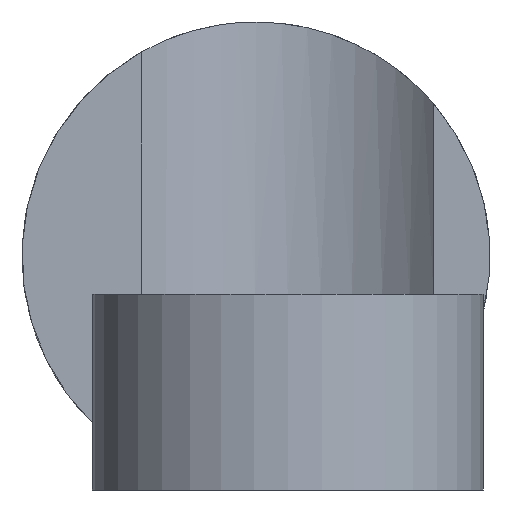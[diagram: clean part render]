
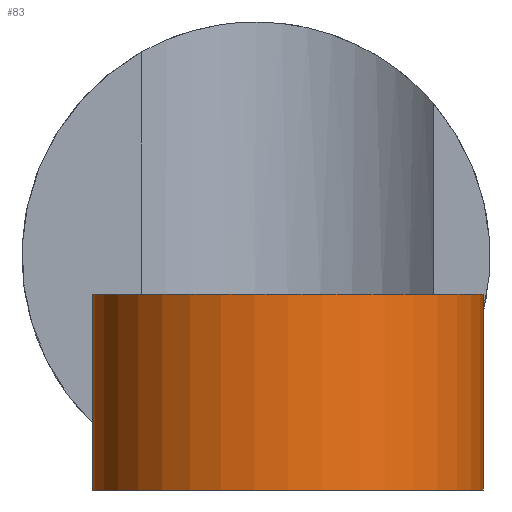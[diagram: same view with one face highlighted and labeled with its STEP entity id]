
A CAD part, left-side view. The second image highlights one B-rep face of the part: STEP entity #83.
In plain terms, the highlighted cylindrical face has radius 6 mm (diameter 12 mm), a partial arc.
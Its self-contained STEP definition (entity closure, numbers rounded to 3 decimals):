
#21 = DIRECTION ( 'NONE',  ( 0., 0., -1. ) ) ;
#33 = DIRECTION ( 'NONE',  ( 0., 0., 1. ) ) ;
#43 = CARTESIAN_POINT ( 'NONE',  ( -17.5, 0., 6. ) ) ;
#61 = ORIENTED_EDGE ( 'NONE', *, *, #650, .F. ) ;
#64 = EDGE_CURVE ( 'NONE', #550, #421, #157, .T. ) ;
#72 = AXIS2_PLACEMENT_3D ( 'NONE', #43, #623, #237 ) ;
#83 = ADVANCED_FACE ( 'NONE', ( #720 ), #537, .T. ) ;
#84 = CARTESIAN_POINT ( 'NONE',  ( -17.5, -6., 0. ) ) ;
#95 = CARTESIAN_POINT ( 'NONE',  ( -17.5, 0., 0. ) ) ;
#115 = CARTESIAN_POINT ( 'NONE',  ( -17.5, 6., 0. ) ) ;
#157 = LINE ( 'NONE', #440, #447 ) ;
#236 = AXIS2_PLACEMENT_3D ( 'NONE', #656, #21, #489 ) ;
#237 = DIRECTION ( 'NONE',  ( -1., 0., 0. ) ) ;
#262 = CIRCLE ( 'NONE', #236, 6. ) ;
#264 = EDGE_CURVE ( 'NONE', #421, #706, #500, .T. ) ;
#285 = VECTOR ( 'NONE', #33, 1000. ) ;
#325 = AXIS2_PLACEMENT_3D ( 'NONE', #95, #665, #496 ) ;
#397 = ORIENTED_EDGE ( 'NONE', *, *, #264, .T. ) ;
#413 = VERTEX_POINT ( 'NONE', #115 ) ;
#421 = VERTEX_POINT ( 'NONE', #530 ) ;
#440 = CARTESIAN_POINT ( 'NONE',  ( -17.5, -6., 0. ) ) ;
#447 = VECTOR ( 'NONE', #609, 1000. ) ;
#489 = DIRECTION ( 'NONE',  ( -1., 0., 0. ) ) ;
#496 = DIRECTION ( 'NONE',  ( 1., 0., 0. ) ) ;
#500 = CIRCLE ( 'NONE', #72, 6. ) ;
#530 = CARTESIAN_POINT ( 'NONE',  ( -17.5, -6., 6. ) ) ;
#534 = CARTESIAN_POINT ( 'NONE',  ( -17.5, 6., 0. ) ) ;
#537 = CYLINDRICAL_SURFACE ( 'NONE', #325, 6. ) ;
#550 = VERTEX_POINT ( 'NONE', #84 ) ;
#555 = EDGE_CURVE ( 'NONE', #550, #413, #262, .T. ) ;
#557 = LINE ( 'NONE', #534, #285 ) ;
#589 = ORIENTED_EDGE ( 'NONE', *, *, #64, .T. ) ;
#609 = DIRECTION ( 'NONE',  ( 0., 0., 1. ) ) ;
#623 = DIRECTION ( 'NONE',  ( 0., 0., -1. ) ) ;
#650 = EDGE_CURVE ( 'NONE', #413, #706, #557, .T. ) ;
#656 = CARTESIAN_POINT ( 'NONE',  ( -17.5, 0., 0. ) ) ;
#663 = ORIENTED_EDGE ( 'NONE', *, *, #555, .F. ) ;
#665 = DIRECTION ( 'NONE',  ( 0., 0., 1. ) ) ;
#696 = EDGE_LOOP ( 'NONE', ( #589, #397, #61, #663 ) ) ;
#706 = VERTEX_POINT ( 'NONE', #722 ) ;
#720 = FACE_OUTER_BOUND ( 'NONE', #696, .T. ) ;
#722 = CARTESIAN_POINT ( 'NONE',  ( -17.5, 6., 6. ) ) ;
